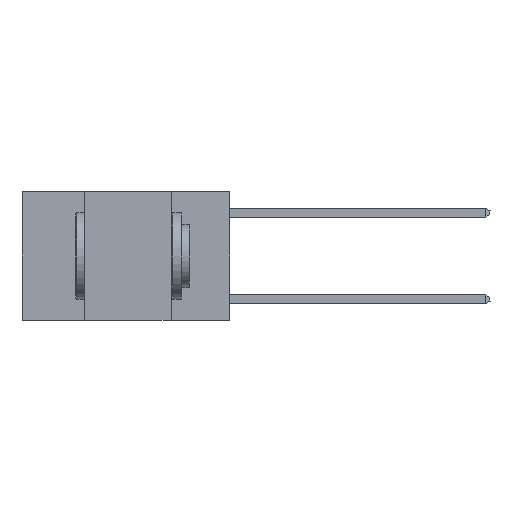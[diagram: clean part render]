
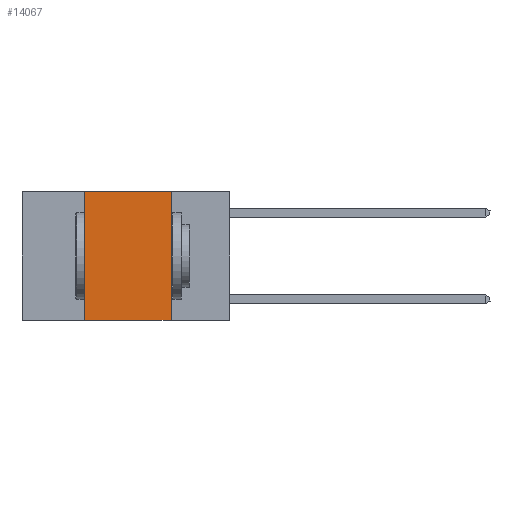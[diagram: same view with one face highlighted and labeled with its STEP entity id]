
A CAD part, left-side view. The second image highlights one B-rep face of the part: STEP entity #14067.
In plain terms, the highlighted planar face has unit normal (-1, 0, 0).
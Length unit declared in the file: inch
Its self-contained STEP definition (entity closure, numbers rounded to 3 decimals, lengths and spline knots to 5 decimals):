
#121 = LINE ( 'NONE', #7628, #11971 ) ;
#2640 = DIRECTION ( 'NONE',  ( 1., 0., 0. ) ) ;
#2659 = CARTESIAN_POINT ( 'NONE',  ( 0., 0.42, 0. ) ) ;
#6002 = VECTOR ( 'NONE', #12372, 39.37008 ) ;
#6534 = VECTOR ( 'NONE', #23618, 39.37008 ) ;
#7107 = VERTEX_POINT ( 'NONE', #28687 ) ;
#7189 = DIRECTION ( 'NONE',  ( 0., -1., 0. ) ) ;
#7628 = CARTESIAN_POINT ( 'NONE',  ( 0., 0.17, 0. ) ) ;
#8296 = VECTOR ( 'NONE', #7189, 39.37008 ) ;
#10491 = ORIENTED_EDGE ( 'NONE', *, *, #24276, .F. ) ;
#11971 = VECTOR ( 'NONE', #20892, 39.37008 ) ;
#12173 = LINE ( 'NONE', #28260, #6534 ) ;
#12240 = EDGE_CURVE ( 'NONE', #24318, #7107, #12173, .T. ) ;
#12345 = VERTEX_POINT ( 'NONE', #19101 ) ;
#12372 = DIRECTION ( 'NONE',  ( 0., 0., 1. ) ) ;
#13246 = AXIS2_PLACEMENT_3D ( 'NONE', #23401, #2640, #28326 ) ;
#13801 = CARTESIAN_POINT ( 'NONE',  ( 0., 0.6, 0. ) ) ;
#14067 = ADVANCED_FACE ( 'NONE', ( #23245 ), #19161, .F. ) ;
#18770 = LINE ( 'NONE', #13801, #8296 ) ;
#19101 = CARTESIAN_POINT ( 'NONE',  ( 0., 0.42, 0. ) ) ;
#19161 = PLANE ( 'NONE',  #13246 ) ;
#20019 = EDGE_LOOP ( 'NONE', ( #27843, #10491, #26495, #24535 ) ) ;
#20446 = EDGE_CURVE ( 'NONE', #28839, #7107, #121, .T. ) ;
#20862 = LINE ( 'NONE', #2659, #6002 ) ;
#20892 = DIRECTION ( 'NONE',  ( 0., 0., -1. ) ) ;
#23245 = FACE_OUTER_BOUND ( 'NONE', #20019, .T. ) ;
#23401 = CARTESIAN_POINT ( 'NONE',  ( 0., 0.6, 0. ) ) ;
#23618 = DIRECTION ( 'NONE',  ( 0., -1., 0. ) ) ;
#23876 = CARTESIAN_POINT ( 'NONE',  ( 0., 0.42, -0.37 ) ) ;
#24276 = EDGE_CURVE ( 'NONE', #12345, #28839, #18770, .T. ) ;
#24318 = VERTEX_POINT ( 'NONE', #23876 ) ;
#24535 = ORIENTED_EDGE ( 'NONE', *, *, #12240, .T. ) ;
#26495 = ORIENTED_EDGE ( 'NONE', *, *, #28643, .F. ) ;
#27843 = ORIENTED_EDGE ( 'NONE', *, *, #20446, .F. ) ;
#28260 = CARTESIAN_POINT ( 'NONE',  ( 0., 0.6, -0.37 ) ) ;
#28326 = DIRECTION ( 'NONE',  ( 0., 0., -1. ) ) ;
#28643 = EDGE_CURVE ( 'NONE', #24318, #12345, #20862, .T. ) ;
#28687 = CARTESIAN_POINT ( 'NONE',  ( 0., 0.17, -0.37 ) ) ;
#28839 = VERTEX_POINT ( 'NONE', #29210 ) ;
#29210 = CARTESIAN_POINT ( 'NONE',  ( 0., 0.17, 0. ) ) ;
